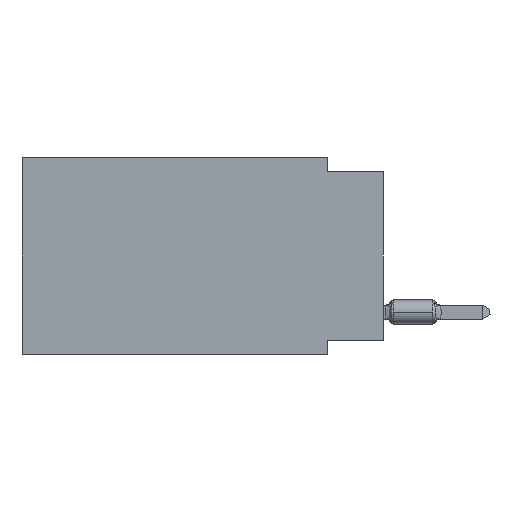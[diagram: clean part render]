
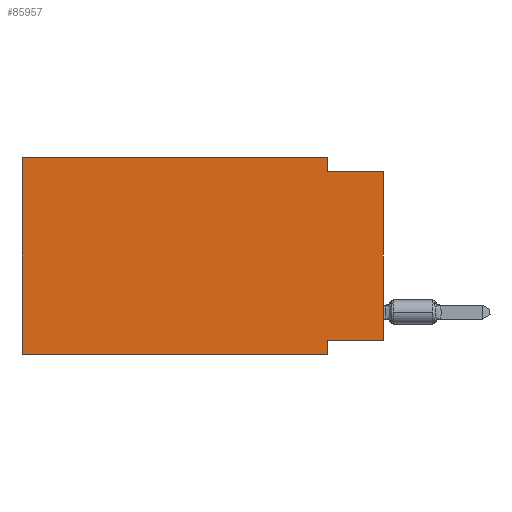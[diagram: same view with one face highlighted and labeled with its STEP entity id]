
A CAD part, left-side view. The second image highlights one B-rep face of the part: STEP entity #85957.
In plain terms, the highlighted planar face has unit normal (-1, 0, 0).
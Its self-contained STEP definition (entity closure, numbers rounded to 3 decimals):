
#1203 = EDGE_CURVE ( 'NONE', #5994, #56270, #49367, .T. ) ;
#1567 = CARTESIAN_POINT ( 'NONE',  ( 0., 2.54, -8.255 ) ) ;
#1897 = CARTESIAN_POINT ( 'NONE',  ( 0., 0., -8.255 ) ) ;
#5994 = VERTEX_POINT ( 'NONE', #41431 ) ;
#6070 = CARTESIAN_POINT ( 'NONE',  ( 0., 16.383, 0. ) ) ;
#8771 = ORIENTED_EDGE ( 'NONE', *, *, #40594, .T. ) ;
#9864 = LINE ( 'NONE', #61314, #25228 ) ;
#10318 = EDGE_LOOP ( 'NONE', ( #8771, #87524, #57053, #27293, #11419, #47275, #53938, #63033 ) ) ;
#11419 = ORIENTED_EDGE ( 'NONE', *, *, #42699, .F. ) ;
#11733 = LINE ( 'NONE', #54087, #66420 ) ;
#11849 = DIRECTION ( 'NONE',  ( 0., 0., -1. ) ) ;
#12018 = VERTEX_POINT ( 'NONE', #80976 ) ;
#12160 = LINE ( 'NONE', #41962, #79315 ) ;
#12794 = EDGE_CURVE ( 'NONE', #54967, #38483, #11733, .T. ) ;
#16655 = CARTESIAN_POINT ( 'NONE',  ( 0., 16.383, 0. ) ) ;
#17125 = DIRECTION ( 'NONE',  ( 0., 0., -1. ) ) ;
#19859 = LINE ( 'NONE', #49675, #65316 ) ;
#21285 = AXIS2_PLACEMENT_3D ( 'NONE', #16655, #68589, #17125 ) ;
#23006 = DIRECTION ( 'NONE',  ( 0., 0., 1. ) ) ;
#24413 = VERTEX_POINT ( 'NONE', #41640 ) ;
#25228 = VECTOR ( 'NONE', #30098, 1000. ) ;
#25337 = CARTESIAN_POINT ( 'NONE',  ( 0., 2.54, 0. ) ) ;
#27293 = ORIENTED_EDGE ( 'NONE', *, *, #51234, .F. ) ;
#29605 = DIRECTION ( 'NONE',  ( 0., -1., 0. ) ) ;
#30098 = DIRECTION ( 'NONE',  ( 0., -1., 0. ) ) ;
#33227 = EDGE_CURVE ( 'NONE', #58366, #12018, #19859, .T. ) ;
#36071 = LINE ( 'NONE', #44227, #92640 ) ;
#37015 = DIRECTION ( 'NONE',  ( 0., 0., -1. ) ) ;
#38483 = VERTEX_POINT ( 'NONE', #1567 ) ;
#38505 = VECTOR ( 'NONE', #23006, 1000. ) ;
#39654 = DIRECTION ( 'NONE',  ( 0., 1., 0. ) ) ;
#40186 = PLANE ( 'NONE',  #21285 ) ;
#40594 = EDGE_CURVE ( 'NONE', #54967, #24413, #74465, .T. ) ;
#41431 = CARTESIAN_POINT ( 'NONE',  ( 0., 2.54, 0. ) ) ;
#41640 = CARTESIAN_POINT ( 'NONE',  ( 0., 0., -0.635 ) ) ;
#41962 = CARTESIAN_POINT ( 'NONE',  ( 0., 16.383, 0. ) ) ;
#42699 = EDGE_CURVE ( 'NONE', #58366, #52829, #12160, .T. ) ;
#44227 = CARTESIAN_POINT ( 'NONE',  ( 0., 2.54, -8.89 ) ) ;
#45192 = VECTOR ( 'NONE', #29605, 1000. ) ;
#45936 = EDGE_CURVE ( 'NONE', #38483, #12018, #36071, .T. ) ;
#47275 = ORIENTED_EDGE ( 'NONE', *, *, #33227, .T. ) ;
#49205 = DIRECTION ( 'NONE',  ( 0., -1., 0. ) ) ;
#49367 = LINE ( 'NONE', #25337, #52439 ) ;
#49675 = CARTESIAN_POINT ( 'NONE',  ( 0., 16.383, -8.89 ) ) ;
#51234 = EDGE_CURVE ( 'NONE', #52829, #5994, #94548, .T. ) ;
#51378 = EDGE_CURVE ( 'NONE', #56270, #24413, #9864, .T. ) ;
#52439 = VECTOR ( 'NONE', #11849, 1000. ) ;
#52787 = CARTESIAN_POINT ( 'NONE',  ( 0., 16.383, -8.89 ) ) ;
#52829 = VERTEX_POINT ( 'NONE', #73825 ) ;
#53938 = ORIENTED_EDGE ( 'NONE', *, *, #45936, .F. ) ;
#54087 = CARTESIAN_POINT ( 'NONE',  ( 0., 0., -8.255 ) ) ;
#54967 = VERTEX_POINT ( 'NONE', #1897 ) ;
#56270 = VERTEX_POINT ( 'NONE', #88603 ) ;
#56886 = DIRECTION ( 'NONE',  ( 0., 0., 1. ) ) ;
#57053 = ORIENTED_EDGE ( 'NONE', *, *, #1203, .F. ) ;
#58366 = VERTEX_POINT ( 'NONE', #52787 ) ;
#61314 = CARTESIAN_POINT ( 'NONE',  ( 0., 0., -0.635 ) ) ;
#63033 = ORIENTED_EDGE ( 'NONE', *, *, #12794, .F. ) ;
#65316 = VECTOR ( 'NONE', #49205, 1000. ) ;
#66420 = VECTOR ( 'NONE', #39654, 1000. ) ;
#68109 = FACE_OUTER_BOUND ( 'NONE', #10318, .T. ) ;
#68589 = DIRECTION ( 'NONE',  ( 1., 0., 0. ) ) ;
#73825 = CARTESIAN_POINT ( 'NONE',  ( 0., 16.383, 0. ) ) ;
#74465 = LINE ( 'NONE', #88879, #38505 ) ;
#79315 = VECTOR ( 'NONE', #56886, 1000. ) ;
#80976 = CARTESIAN_POINT ( 'NONE',  ( 0., 2.54, -8.89 ) ) ;
#85957 = ADVANCED_FACE ( 'NONE', ( #68109 ), #40186, .F. ) ;
#87524 = ORIENTED_EDGE ( 'NONE', *, *, #51378, .F. ) ;
#88603 = CARTESIAN_POINT ( 'NONE',  ( 0., 2.54, -0.635 ) ) ;
#88879 = CARTESIAN_POINT ( 'NONE',  ( 0., 0., 0. ) ) ;
#92640 = VECTOR ( 'NONE', #37015, 1000. ) ;
#94548 = LINE ( 'NONE', #6070, #45192 ) ;
